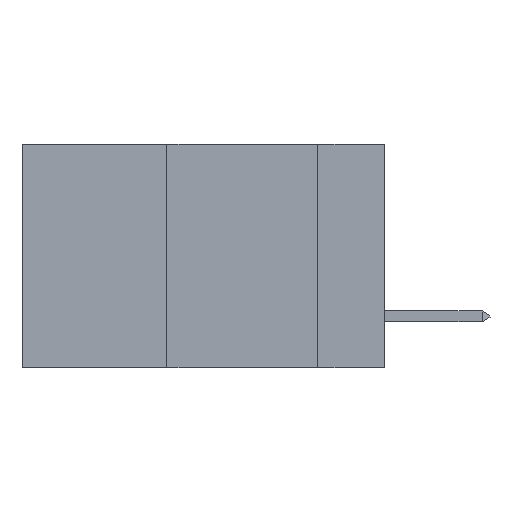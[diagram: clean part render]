
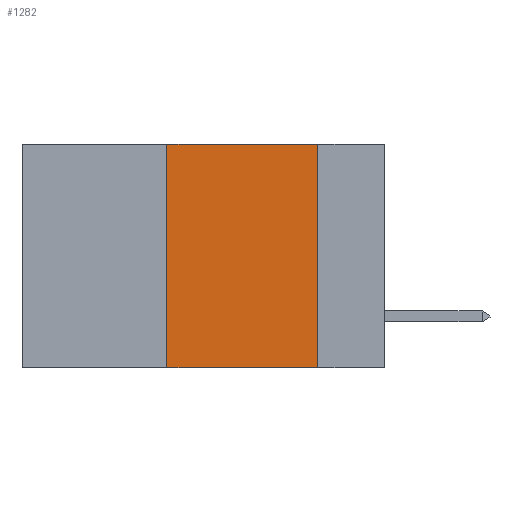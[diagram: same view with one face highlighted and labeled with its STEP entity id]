
A CAD part, left-side view. The second image highlights one B-rep face of the part: STEP entity #1282.
In plain terms, the highlighted planar face has unit normal (-1, 0, 0).
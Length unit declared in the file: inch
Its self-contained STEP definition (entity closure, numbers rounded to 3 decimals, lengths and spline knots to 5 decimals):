
#486 = VECTOR ( 'NONE', #5073, 39.37008 ) ;
#659 = DIRECTION ( 'NONE',  ( 0., 0., 1. ) ) ;
#794 = LINE ( 'NONE', #7992, #2705 ) ;
#1282 = ADVANCED_FACE ( 'NONE', ( #9511 ), #3270, .F. ) ;
#1290 = CARTESIAN_POINT ( 'NONE',  ( 0., 0.36, 0. ) ) ;
#1885 = DIRECTION ( 'NONE',  ( 0., 0., -1. ) ) ;
#2115 = CARTESIAN_POINT ( 'NONE',  ( 0., 0.6, 0. ) ) ;
#2161 = EDGE_LOOP ( 'NONE', ( #7073, #3320, #8585, #8832 ) ) ;
#2253 = VECTOR ( 'NONE', #659, 39.37008 ) ;
#2705 = VECTOR ( 'NONE', #3678, 39.37008 ) ;
#3270 = PLANE ( 'NONE',  #5326 ) ;
#3320 = ORIENTED_EDGE ( 'NONE', *, *, #3925, .F. ) ;
#3645 = VERTEX_POINT ( 'NONE', #5196 ) ;
#3678 = DIRECTION ( 'NONE',  ( 0., -1., 0. ) ) ;
#3925 = EDGE_CURVE ( 'NONE', #4504, #7001, #794, .T. ) ;
#4009 = VERTEX_POINT ( 'NONE', #8352 ) ;
#4254 = DIRECTION ( 'NONE',  ( 0., 0., -1. ) ) ;
#4504 = VERTEX_POINT ( 'NONE', #1290 ) ;
#5026 = EDGE_CURVE ( 'NONE', #3645, #4009, #8568, .T. ) ;
#5073 = DIRECTION ( 'NONE',  ( 0., -1., 0. ) ) ;
#5122 = CARTESIAN_POINT ( 'NONE',  ( 0., 0.11, 0. ) ) ;
#5196 = CARTESIAN_POINT ( 'NONE',  ( 0., 0.36, -0.37 ) ) ;
#5326 = AXIS2_PLACEMENT_3D ( 'NONE', #2115, #5415, #4254 ) ;
#5415 = DIRECTION ( 'NONE',  ( 1., 0., 0. ) ) ;
#5494 = CARTESIAN_POINT ( 'NONE',  ( 0., 0.36, 0. ) ) ;
#6521 = CARTESIAN_POINT ( 'NONE',  ( 0., 0.11, 0. ) ) ;
#6921 = VECTOR ( 'NONE', #1885, 39.37008 ) ;
#7001 = VERTEX_POINT ( 'NONE', #5122 ) ;
#7051 = CARTESIAN_POINT ( 'NONE',  ( 0., 0.6, -0.37 ) ) ;
#7067 = EDGE_CURVE ( 'NONE', #3645, #4504, #8416, .T. ) ;
#7073 = ORIENTED_EDGE ( 'NONE', *, *, #8397, .F. ) ;
#7992 = CARTESIAN_POINT ( 'NONE',  ( 0., 0.6, 0. ) ) ;
#8352 = CARTESIAN_POINT ( 'NONE',  ( 0., 0.11, -0.37 ) ) ;
#8397 = EDGE_CURVE ( 'NONE', #7001, #4009, #8699, .T. ) ;
#8416 = LINE ( 'NONE', #5494, #2253 ) ;
#8568 = LINE ( 'NONE', #7051, #486 ) ;
#8585 = ORIENTED_EDGE ( 'NONE', *, *, #7067, .F. ) ;
#8699 = LINE ( 'NONE', #6521, #6921 ) ;
#8832 = ORIENTED_EDGE ( 'NONE', *, *, #5026, .T. ) ;
#9511 = FACE_OUTER_BOUND ( 'NONE', #2161, .T. ) ;
